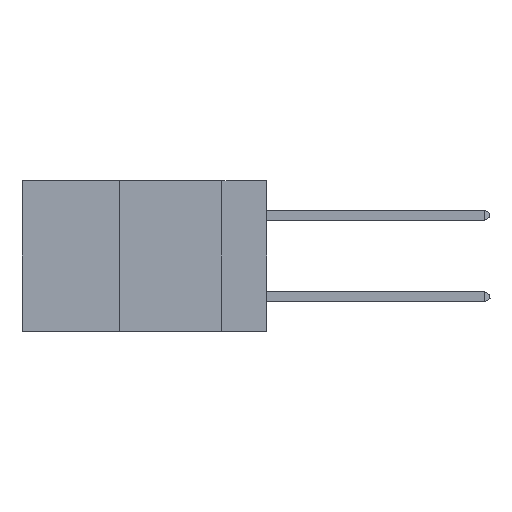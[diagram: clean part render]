
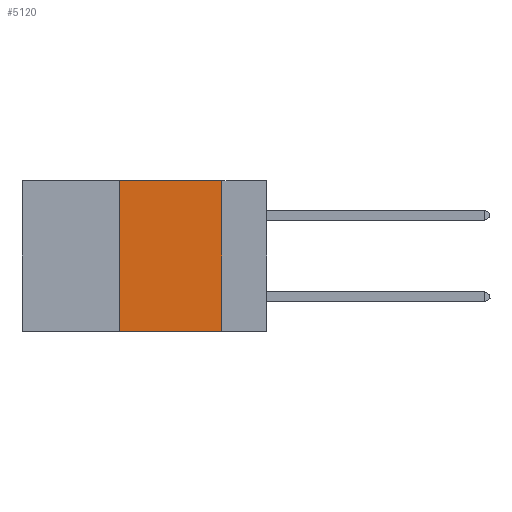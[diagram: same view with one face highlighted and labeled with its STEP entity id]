
A CAD part, left-side view. The second image highlights one B-rep face of the part: STEP entity #5120.
In plain terms, the highlighted planar face has unit normal (-1, 0, 0).
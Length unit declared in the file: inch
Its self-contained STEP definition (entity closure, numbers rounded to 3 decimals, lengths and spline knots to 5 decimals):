
#1332 = CARTESIAN_POINT ( 'NONE',  ( 0., 0.36, -0.37 ) ) ;
#1379 = CARTESIAN_POINT ( 'NONE',  ( 0., 0.36, 0. ) ) ;
#2065 = ORIENTED_EDGE ( 'NONE', *, *, #21035, .F. ) ;
#3137 = ORIENTED_EDGE ( 'NONE', *, *, #6078, .F. ) ;
#3678 = LINE ( 'NONE', #18694, #7085 ) ;
#3699 = CARTESIAN_POINT ( 'NONE',  ( 0., 0.6, 0. ) ) ;
#5120 = ADVANCED_FACE ( 'NONE', ( #13281 ), #19332, .F. ) ;
#5390 = EDGE_CURVE ( 'NONE', #20333, #21324, #8932, .T. ) ;
#5781 = DIRECTION ( 'NONE',  ( 0., 0., 1. ) ) ;
#5919 = VECTOR ( 'NONE', #9991, 39.37008 ) ;
#6078 = EDGE_CURVE ( 'NONE', #25494, #21842, #6912, .T. ) ;
#6912 = LINE ( 'NONE', #3699, #20997 ) ;
#7085 = VECTOR ( 'NONE', #27529, 39.37008 ) ;
#7324 = DIRECTION ( 'NONE',  ( 0., -1., 0. ) ) ;
#8888 = DIRECTION ( 'NONE',  ( 1., 0., 0. ) ) ;
#8932 = LINE ( 'NONE', #25255, #5919 ) ;
#9991 = DIRECTION ( 'NONE',  ( 0., -1., 0. ) ) ;
#13281 = FACE_OUTER_BOUND ( 'NONE', #19683, .T. ) ;
#17248 = CARTESIAN_POINT ( 'NONE',  ( 0., 0.6, 0. ) ) ;
#18674 = CARTESIAN_POINT ( 'NONE',  ( 0., 0.36, 0. ) ) ;
#18694 = CARTESIAN_POINT ( 'NONE',  ( 0., 0.11, 0. ) ) ;
#19332 = PLANE ( 'NONE',  #20348 ) ;
#19568 = CARTESIAN_POINT ( 'NONE',  ( 0., 0.11, -0.37 ) ) ;
#19683 = EDGE_LOOP ( 'NONE', ( #22899, #3137, #2065, #23780 ) ) ;
#20333 = VERTEX_POINT ( 'NONE', #1332 ) ;
#20348 = AXIS2_PLACEMENT_3D ( 'NONE', #17248, #8888, #23848 ) ;
#20997 = VECTOR ( 'NONE', #7324, 39.37008 ) ;
#21035 = EDGE_CURVE ( 'NONE', #20333, #25494, #26568, .T. ) ;
#21197 = VECTOR ( 'NONE', #5781, 39.37008 ) ;
#21324 = VERTEX_POINT ( 'NONE', #19568 ) ;
#21842 = VERTEX_POINT ( 'NONE', #23513 ) ;
#22899 = ORIENTED_EDGE ( 'NONE', *, *, #25585, .F. ) ;
#23513 = CARTESIAN_POINT ( 'NONE',  ( 0., 0.11, 0. ) ) ;
#23780 = ORIENTED_EDGE ( 'NONE', *, *, #5390, .T. ) ;
#23848 = DIRECTION ( 'NONE',  ( 0., 0., -1. ) ) ;
#25255 = CARTESIAN_POINT ( 'NONE',  ( 0., 0.6, -0.37 ) ) ;
#25494 = VERTEX_POINT ( 'NONE', #1379 ) ;
#25585 = EDGE_CURVE ( 'NONE', #21842, #21324, #3678, .T. ) ;
#26568 = LINE ( 'NONE', #18674, #21197 ) ;
#27529 = DIRECTION ( 'NONE',  ( 0., 0., -1. ) ) ;
